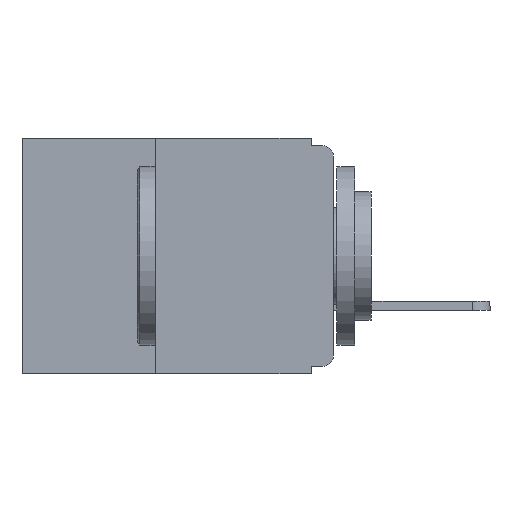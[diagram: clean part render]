
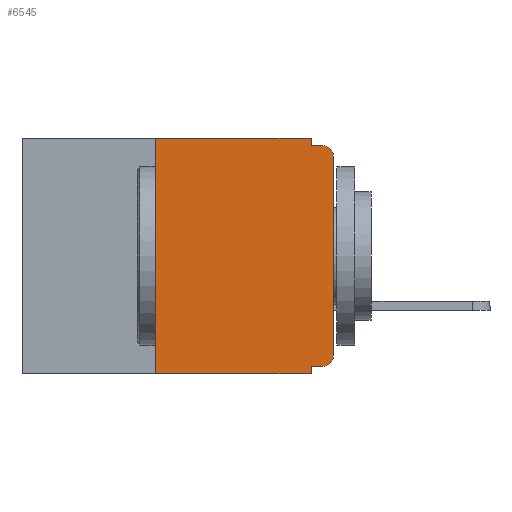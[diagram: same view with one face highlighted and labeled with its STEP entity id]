
A CAD part, left-side view. The second image highlights one B-rep face of the part: STEP entity #6545.
In plain terms, the highlighted planar face has unit normal (-1, 0, 0).
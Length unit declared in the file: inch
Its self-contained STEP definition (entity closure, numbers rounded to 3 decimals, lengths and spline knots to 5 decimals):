
#584 = CARTESIAN_POINT ( 'NONE',  ( 0., 0.25, 0. ) ) ;
#739 = CARTESIAN_POINT ( 'NONE',  ( 0., 0.437, -0.33 ) ) ;
#758 = ORIENTED_EDGE ( 'NONE', *, *, #9908, .T. ) ;
#930 = VERTEX_POINT ( 'NONE', #16691 ) ;
#988 = AXIS2_PLACEMENT_3D ( 'NONE', #22545, #9253, #24746 ) ;
#1039 = CARTESIAN_POINT ( 'NONE',  ( 0., 0.031, -0.33 ) ) ;
#1374 = LINE ( 'NONE', #27302, #7265 ) ;
#2449 = LINE ( 'NONE', #26296, #25340 ) ;
#2934 = FACE_OUTER_BOUND ( 'NONE', #8922, .T. ) ;
#2936 = DIRECTION ( 'NONE',  ( 0., 0., 1. ) ) ;
#2941 = LINE ( 'NONE', #1039, #19984 ) ;
#3133 = VERTEX_POINT ( 'NONE', #11305 ) ;
#3260 = DIRECTION ( 'NONE',  ( 0., 0., -1. ) ) ;
#3264 = CARTESIAN_POINT ( 'NONE',  ( 0., 0., -0.32 ) ) ;
#3968 = VECTOR ( 'NONE', #10250, 39.37008 ) ;
#4035 = CARTESIAN_POINT ( 'NONE',  ( 0., 0.015, -0.32 ) ) ;
#4739 = ORIENTED_EDGE ( 'NONE', *, *, #12842, .F. ) ;
#5051 = VECTOR ( 'NONE', #11782, 39.37008 ) ;
#5275 = EDGE_CURVE ( 'NONE', #8983, #18818, #6845, .T. ) ;
#6222 = VERTEX_POINT ( 'NONE', #18524 ) ;
#6375 = CARTESIAN_POINT ( 'NONE',  ( 0., 0.437, 0. ) ) ;
#6545 = ADVANCED_FACE ( 'NONE', ( #2934 ), #19686, .F. ) ;
#6573 = AXIS2_PLACEMENT_3D ( 'NONE', #22210, #8897, #24410 ) ;
#6607 = ORIENTED_EDGE ( 'NONE', *, *, #7819, .F. ) ;
#6608 = LINE ( 'NONE', #27205, #11821 ) ;
#6845 = LINE ( 'NONE', #26372, #23164 ) ;
#7265 = VECTOR ( 'NONE', #20734, 39.37008 ) ;
#7819 = EDGE_CURVE ( 'NONE', #18818, #10477, #26797, .T. ) ;
#8218 = EDGE_CURVE ( 'NONE', #930, #10477, #11218, .T. ) ;
#8596 = DIRECTION ( 'NONE',  ( 0., 0., -1. ) ) ;
#8741 = AXIS2_PLACEMENT_3D ( 'NONE', #6375, #21904, #8596 ) ;
#8897 = DIRECTION ( 'NONE',  ( -1., 0., 0. ) ) ;
#8898 = ORIENTED_EDGE ( 'NONE', *, *, #28307, .T. ) ;
#8922 = EDGE_LOOP ( 'NONE', ( #8898, #28449, #6607, #14346, #4739, #16811, #17601, #12553, #18158, #758 ) ) ;
#8983 = VERTEX_POINT ( 'NONE', #25189 ) ;
#9253 = DIRECTION ( 'NONE',  ( -1., 0., 0. ) ) ;
#9641 = EDGE_CURVE ( 'NONE', #6222, #9855, #2941, .T. ) ;
#9855 = VERTEX_POINT ( 'NONE', #28163 ) ;
#9908 = EDGE_CURVE ( 'NONE', #23927, #3133, #13709, .T. ) ;
#10250 = DIRECTION ( 'NONE',  ( 0., -1., 0. ) ) ;
#10477 = VERTEX_POINT ( 'NONE', #26293 ) ;
#11218 = CIRCLE ( 'NONE', #988, 0.015 ) ;
#11305 = CARTESIAN_POINT ( 'NONE',  ( 0., 0., -0.305 ) ) ;
#11782 = DIRECTION ( 'NONE',  ( 0., -1., 0. ) ) ;
#11821 = VECTOR ( 'NONE', #2936, 39.37008 ) ;
#12046 = EDGE_CURVE ( 'NONE', #23927, #6222, #21582, .T. ) ;
#12512 = CARTESIAN_POINT ( 'NONE',  ( 0., 0., -0.01 ) ) ;
#12553 = ORIENTED_EDGE ( 'NONE', *, *, #9641, .F. ) ;
#12842 = EDGE_CURVE ( 'NONE', #26301, #8983, #1374, .T. ) ;
#13709 = CIRCLE ( 'NONE', #6573, 0.015 ) ;
#14346 = ORIENTED_EDGE ( 'NONE', *, *, #5275, .F. ) ;
#16691 = CARTESIAN_POINT ( 'NONE',  ( 0., 0., -0.025 ) ) ;
#16811 = ORIENTED_EDGE ( 'NONE', *, *, #28563, .F. ) ;
#17601 = ORIENTED_EDGE ( 'NONE', *, *, #19811, .T. ) ;
#18158 = ORIENTED_EDGE ( 'NONE', *, *, #12046, .F. ) ;
#18524 = CARTESIAN_POINT ( 'NONE',  ( 0., 0.031, -0.32 ) ) ;
#18792 = DIRECTION ( 'NONE',  ( 0., 1., 0. ) ) ;
#18818 = VERTEX_POINT ( 'NONE', #23961 ) ;
#19686 = PLANE ( 'NONE',  #8741 ) ;
#19770 = DIRECTION ( 'NONE',  ( 0., 0., 1. ) ) ;
#19811 = EDGE_CURVE ( 'NONE', #19880, #9855, #23476, .T. ) ;
#19880 = VERTEX_POINT ( 'NONE', #27493 ) ;
#19984 = VECTOR ( 'NONE', #3260, 39.37008 ) ;
#20734 = DIRECTION ( 'NONE',  ( 0., -1., 0. ) ) ;
#21582 = LINE ( 'NONE', #3264, #27348 ) ;
#21904 = DIRECTION ( 'NONE',  ( 1., 0., 0. ) ) ;
#22210 = CARTESIAN_POINT ( 'NONE',  ( 0., 0.015, -0.305 ) ) ;
#22545 = CARTESIAN_POINT ( 'NONE',  ( 0., 0.015, -0.025 ) ) ;
#23164 = VECTOR ( 'NONE', #28531, 39.37008 ) ;
#23476 = LINE ( 'NONE', #739, #5051 ) ;
#23927 = VERTEX_POINT ( 'NONE', #4035 ) ;
#23961 = CARTESIAN_POINT ( 'NONE',  ( 0., 0.031, -0.01 ) ) ;
#24410 = DIRECTION ( 'NONE',  ( 0., 0., -1. ) ) ;
#24746 = DIRECTION ( 'NONE',  ( 0., 0., -1. ) ) ;
#25189 = CARTESIAN_POINT ( 'NONE',  ( 0., 0.031, 0. ) ) ;
#25340 = VECTOR ( 'NONE', #19770, 39.37008 ) ;
#26293 = CARTESIAN_POINT ( 'NONE',  ( 0., 0.015, -0.01 ) ) ;
#26296 = CARTESIAN_POINT ( 'NONE',  ( 0., 0., 0. ) ) ;
#26301 = VERTEX_POINT ( 'NONE', #584 ) ;
#26372 = CARTESIAN_POINT ( 'NONE',  ( 0., 0.031, 0. ) ) ;
#26797 = LINE ( 'NONE', #12512, #3968 ) ;
#27205 = CARTESIAN_POINT ( 'NONE',  ( 0., 0.25, -0.33 ) ) ;
#27302 = CARTESIAN_POINT ( 'NONE',  ( 0., 0.437, 0. ) ) ;
#27348 = VECTOR ( 'NONE', #18792, 39.37008 ) ;
#27493 = CARTESIAN_POINT ( 'NONE',  ( 0., 0.25, -0.33 ) ) ;
#28163 = CARTESIAN_POINT ( 'NONE',  ( 0., 0.031, -0.33 ) ) ;
#28307 = EDGE_CURVE ( 'NONE', #3133, #930, #2449, .T. ) ;
#28449 = ORIENTED_EDGE ( 'NONE', *, *, #8218, .T. ) ;
#28531 = DIRECTION ( 'NONE',  ( 0., 0., -1. ) ) ;
#28563 = EDGE_CURVE ( 'NONE', #19880, #26301, #6608, .T. ) ;
